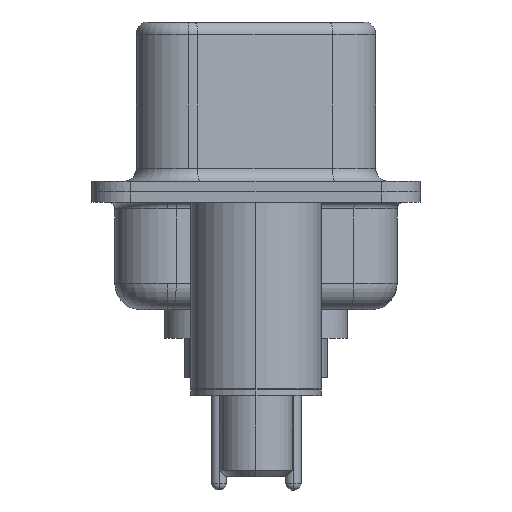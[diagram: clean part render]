
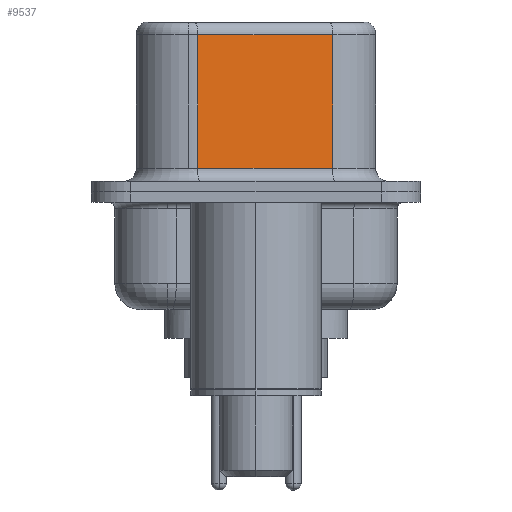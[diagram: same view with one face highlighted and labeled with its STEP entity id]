
A CAD part, left-side view. The second image highlights one B-rep face of the part: STEP entity #9537.
In plain terms, the highlighted planar face has unit normal (-0.985, -0.174, 0).
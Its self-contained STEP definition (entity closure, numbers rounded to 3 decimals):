
#216 = CARTESIAN_POINT ( 'NONE',  ( 4.585, -2.927, 6.52 ) ) ;
#288 = ORIENTED_EDGE ( 'NONE', *, *, #10710, .T. ) ;
#1467 = FACE_OUTER_BOUND ( 'NONE', #3506, .T. ) ;
#2445 = ORIENTED_EDGE ( 'NONE', *, *, #6228, .T. ) ;
#3506 = EDGE_LOOP ( 'NONE', ( #10995, #5586, #2445, #288 ) ) ;
#3613 = EDGE_CURVE ( 'NONE', #6143, #16538, #21011, .T. ) ;
#4640 = EDGE_CURVE ( 'NONE', #6143, #5351, #16338, .T. ) ;
#5003 = VECTOR ( 'NONE', #6524, 1000. ) ;
#5351 = VERTEX_POINT ( 'NONE', #16786 ) ;
#5586 = ORIENTED_EDGE ( 'NONE', *, *, #4640, .T. ) ;
#6143 = VERTEX_POINT ( 'NONE', #13720 ) ;
#6228 = EDGE_CURVE ( 'NONE', #5351, #8256, #6244, .T. ) ;
#6244 = LINE ( 'NONE', #6897, #22508 ) ;
#6524 = DIRECTION ( 'NONE',  ( 0.174, -0.985, 0. ) ) ;
#6586 = VECTOR ( 'NONE', #7969, 1000. ) ;
#6763 = DIRECTION ( 'NONE',  ( 0., 0., -1. ) ) ;
#6773 = CARTESIAN_POINT ( 'NONE',  ( 4.585, -2.927, 0.9 ) ) ;
#6897 = CARTESIAN_POINT ( 'NONE',  ( 3.675, 2.233, 6.52 ) ) ;
#7969 = DIRECTION ( 'NONE',  ( -0.174, 0.985, 0. ) ) ;
#8256 = VERTEX_POINT ( 'NONE', #17825 ) ;
#8313 = VECTOR ( 'NONE', #20974, 1000. ) ;
#8967 = CARTESIAN_POINT ( 'NONE',  ( 4.585, -2.927, 6.02 ) ) ;
#9486 = DIRECTION ( 'NONE',  ( 0.985, 0.174, 0. ) ) ;
#9537 = ADVANCED_FACE ( 'NONE', ( #1467 ), #19784, .F. ) ;
#9709 = LINE ( 'NONE', #18625, #5003 ) ;
#10710 = EDGE_CURVE ( 'NONE', #8256, #16538, #9709, .T. ) ;
#10995 = ORIENTED_EDGE ( 'NONE', *, *, #3613, .F. ) ;
#13155 = AXIS2_PLACEMENT_3D ( 'NONE', #14618, #9486, #21551 ) ;
#13720 = CARTESIAN_POINT ( 'NONE',  ( 4.585, -2.927, 6.02 ) ) ;
#14618 = CARTESIAN_POINT ( 'NONE',  ( 4.585, -2.927, 6.52 ) ) ;
#16338 = LINE ( 'NONE', #8967, #6586 ) ;
#16538 = VERTEX_POINT ( 'NONE', #6773 ) ;
#16786 = CARTESIAN_POINT ( 'NONE',  ( 3.675, 2.233, 6.02 ) ) ;
#17825 = CARTESIAN_POINT ( 'NONE',  ( 3.675, 2.233, 0.9 ) ) ;
#18625 = CARTESIAN_POINT ( 'NONE',  ( 4.585, -2.927, 0.9 ) ) ;
#19784 = PLANE ( 'NONE',  #13155 ) ;
#20974 = DIRECTION ( 'NONE',  ( 0., 0., -1. ) ) ;
#21011 = LINE ( 'NONE', #216, #8313 ) ;
#21551 = DIRECTION ( 'NONE',  ( -0.174, 0.985, 0. ) ) ;
#22508 = VECTOR ( 'NONE', #6763, 1000. ) ;
